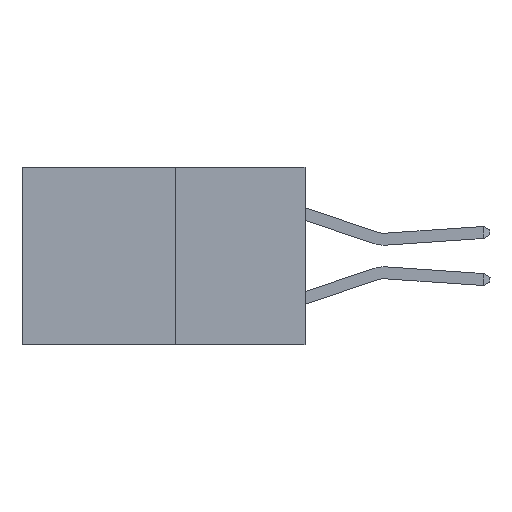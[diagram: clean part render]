
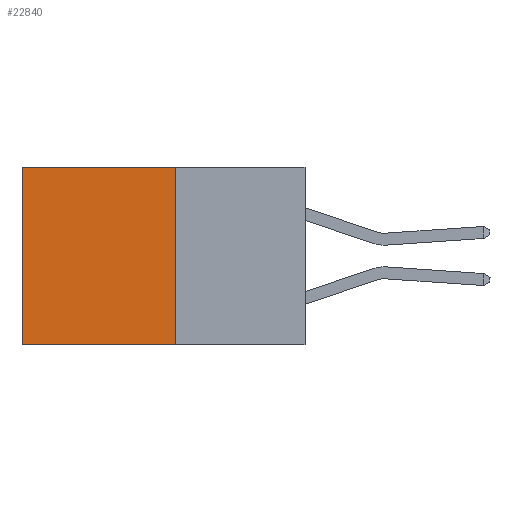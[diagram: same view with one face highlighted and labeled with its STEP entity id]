
A CAD part, left-side view. The second image highlights one B-rep face of the part: STEP entity #22840.
In plain terms, the highlighted planar face has unit normal (-1, 0, 0).
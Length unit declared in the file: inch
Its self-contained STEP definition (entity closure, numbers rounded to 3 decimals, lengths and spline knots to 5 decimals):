
#996 = VECTOR ( 'NONE', #11906, 39.37008 ) ;
#1157 = AXIS2_PLACEMENT_3D ( 'NONE', #5052, #6980, #20170 ) ;
#1883 = VERTEX_POINT ( 'NONE', #7444 ) ;
#2054 = ORIENTED_EDGE ( 'NONE', *, *, #19512, .T. ) ;
#2547 = VECTOR ( 'NONE', #17942, 39.37008 ) ;
#2657 = CARTESIAN_POINT ( 'NONE',  ( 0.277, 0.27, -0.37 ) ) ;
#3464 = EDGE_CURVE ( 'NONE', #11129, #1883, #16220, .T. ) ;
#3670 = FACE_OUTER_BOUND ( 'NONE', #18389, .T. ) ;
#3944 = VECTOR ( 'NONE', #16960, 39.37008 ) ;
#5052 = CARTESIAN_POINT ( 'NONE',  ( 0.277, 0.27, -0.37 ) ) ;
#5678 = CARTESIAN_POINT ( 'NONE',  ( 0.277, 0.59, -0.37 ) ) ;
#6980 = DIRECTION ( 'NONE',  ( 1., 0., 0. ) ) ;
#7444 = CARTESIAN_POINT ( 'NONE',  ( 0.277, 0.59, -0.37 ) ) ;
#7946 = VERTEX_POINT ( 'NONE', #9427 ) ;
#9400 = ORIENTED_EDGE ( 'NONE', *, *, #23700, .F. ) ;
#9427 = CARTESIAN_POINT ( 'NONE',  ( 0.277, 0.27, 0. ) ) ;
#10170 = ORIENTED_EDGE ( 'NONE', *, *, #10283, .F. ) ;
#10283 = EDGE_CURVE ( 'NONE', #23398, #1883, #12665, .T. ) ;
#10435 = ORIENTED_EDGE ( 'NONE', *, *, #3464, .T. ) ;
#10854 = CARTESIAN_POINT ( 'NONE',  ( 0.277, 0.59, 0. ) ) ;
#11129 = VERTEX_POINT ( 'NONE', #10854 ) ;
#11906 = DIRECTION ( 'NONE',  ( 0., 0., -1. ) ) ;
#12665 = LINE ( 'NONE', #2657, #2547 ) ;
#12827 = DIRECTION ( 'NONE',  ( 0., 1., 0. ) ) ;
#13632 = VECTOR ( 'NONE', #12827, 39.37008 ) ;
#14213 = LINE ( 'NONE', #22161, #13632 ) ;
#16220 = LINE ( 'NONE', #5678, #996 ) ;
#16426 = PLANE ( 'NONE',  #1157 ) ;
#16960 = DIRECTION ( 'NONE',  ( 0., 0., -1. ) ) ;
#17942 = DIRECTION ( 'NONE',  ( 0., 1., 0. ) ) ;
#18389 = EDGE_LOOP ( 'NONE', ( #10435, #10170, #9400, #2054 ) ) ;
#18771 = CARTESIAN_POINT ( 'NONE',  ( 0.277, 0.27, -0.37 ) ) ;
#19512 = EDGE_CURVE ( 'NONE', #7946, #11129, #14213, .T. ) ;
#19627 = LINE ( 'NONE', #18771, #3944 ) ;
#20170 = DIRECTION ( 'NONE',  ( 0., 0., -1. ) ) ;
#21668 = CARTESIAN_POINT ( 'NONE',  ( 0.277, 0.27, -0.37 ) ) ;
#22161 = CARTESIAN_POINT ( 'NONE',  ( 0.277, 0.27, 0. ) ) ;
#22840 = ADVANCED_FACE ( 'NONE', ( #3670 ), #16426, .F. ) ;
#23398 = VERTEX_POINT ( 'NONE', #21668 ) ;
#23700 = EDGE_CURVE ( 'NONE', #7946, #23398, #19627, .T. ) ;
